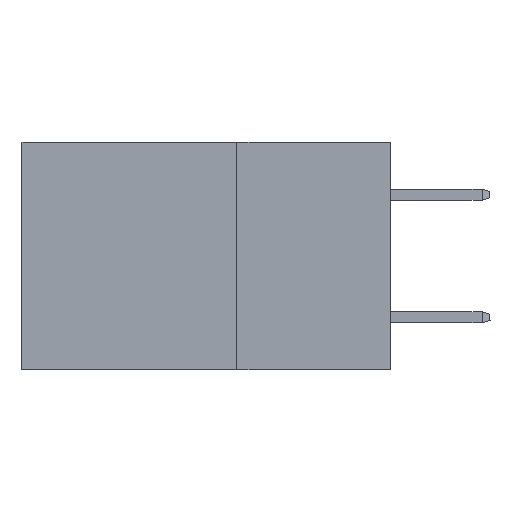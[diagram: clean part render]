
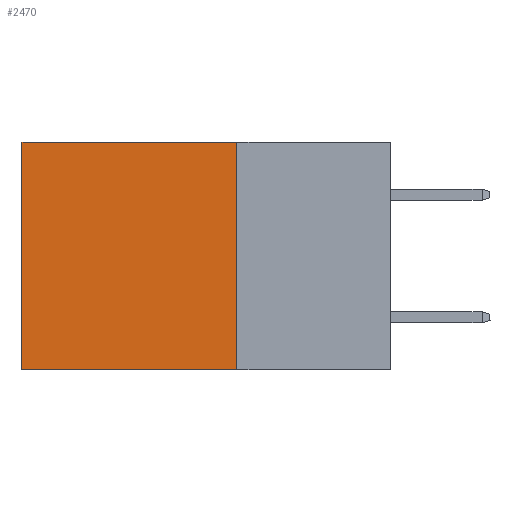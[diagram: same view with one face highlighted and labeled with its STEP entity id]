
A CAD part, left-side view. The second image highlights one B-rep face of the part: STEP entity #2470.
In plain terms, the highlighted planar face has unit normal (-1, 0, 0).
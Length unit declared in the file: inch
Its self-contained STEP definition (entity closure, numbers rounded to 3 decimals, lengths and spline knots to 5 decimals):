
#2470 = ADVANCED_FACE ( 'NONE', ( #44035 ), #36945, .F. ) ;
#2829 = EDGE_CURVE ( 'NONE', #5386, #38800, #24704, .T. ) ;
#4840 = CARTESIAN_POINT ( 'NONE',  ( 0.2875, 0.25, -0.37 ) ) ;
#5386 = VERTEX_POINT ( 'NONE', #4840 ) ;
#6182 = EDGE_CURVE ( 'NONE', #25312, #38800, #25718, .T. ) ;
#10024 = EDGE_LOOP ( 'NONE', ( #32317, #30189, #44286, #42143 ) ) ;
#12220 = DIRECTION ( 'NONE',  ( 0., 0., -1. ) ) ;
#14936 = LINE ( 'NONE', #17677, #22017 ) ;
#17677 = CARTESIAN_POINT ( 'NONE',  ( 0.2875, 0.25, 0. ) ) ;
#17781 = EDGE_CURVE ( 'NONE', #20621, #5386, #14936, .T. ) ;
#18479 = EDGE_CURVE ( 'NONE', #20621, #25312, #21974, .T. ) ;
#19788 = DIRECTION ( 'NONE',  ( 0., 0., -1. ) ) ;
#20621 = VERTEX_POINT ( 'NONE', #31054 ) ;
#21284 = CARTESIAN_POINT ( 'NONE',  ( 0.2875, 0.25, -0.37 ) ) ;
#21974 = LINE ( 'NONE', #43006, #29362 ) ;
#22017 = VECTOR ( 'NONE', #24769, 39.37008 ) ;
#24704 = LINE ( 'NONE', #21284, #37074 ) ;
#24769 = DIRECTION ( 'NONE',  ( 0., 0., -1. ) ) ;
#25312 = VERTEX_POINT ( 'NONE', #40420 ) ;
#25718 = LINE ( 'NONE', #43559, #26140 ) ;
#26140 = VECTOR ( 'NONE', #12220, 39.37008 ) ;
#29362 = VECTOR ( 'NONE', #35922, 39.37008 ) ;
#30189 = ORIENTED_EDGE ( 'NONE', *, *, #2829, .F. ) ;
#30742 = CARTESIAN_POINT ( 'NONE',  ( 0.2875, 0.25, 0. ) ) ;
#31054 = CARTESIAN_POINT ( 'NONE',  ( 0.2875, 0.25, 0. ) ) ;
#31341 = DIRECTION ( 'NONE',  ( 0., 1., 0. ) ) ;
#32317 = ORIENTED_EDGE ( 'NONE', *, *, #6182, .T. ) ;
#35922 = DIRECTION ( 'NONE',  ( 0., 1., 0. ) ) ;
#36908 = CARTESIAN_POINT ( 'NONE',  ( 0.2875, 0.6, -0.37 ) ) ;
#36945 = PLANE ( 'NONE',  #40734 ) ;
#37074 = VECTOR ( 'NONE', #31341, 39.37008 ) ;
#38800 = VERTEX_POINT ( 'NONE', #36908 ) ;
#40420 = CARTESIAN_POINT ( 'NONE',  ( 0.2875, 0.6, 0. ) ) ;
#40734 = AXIS2_PLACEMENT_3D ( 'NONE', #30742, #44699, #19788 ) ;
#42143 = ORIENTED_EDGE ( 'NONE', *, *, #18479, .T. ) ;
#43006 = CARTESIAN_POINT ( 'NONE',  ( 0.2875, 0.25, 0. ) ) ;
#43559 = CARTESIAN_POINT ( 'NONE',  ( 0.2875, 0.6, 0. ) ) ;
#44035 = FACE_OUTER_BOUND ( 'NONE', #10024, .T. ) ;
#44286 = ORIENTED_EDGE ( 'NONE', *, *, #17781, .F. ) ;
#44699 = DIRECTION ( 'NONE',  ( 1., 0., 0. ) ) ;
